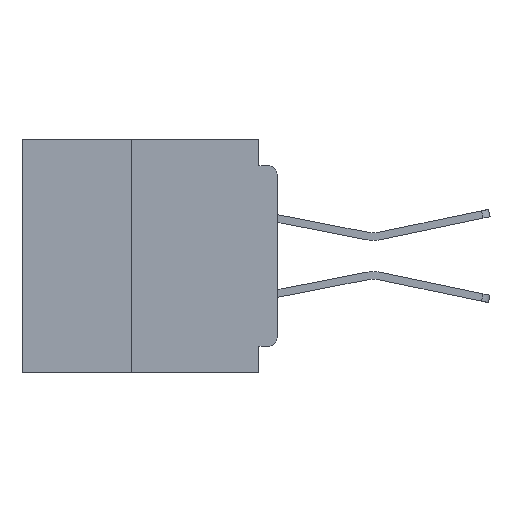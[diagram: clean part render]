
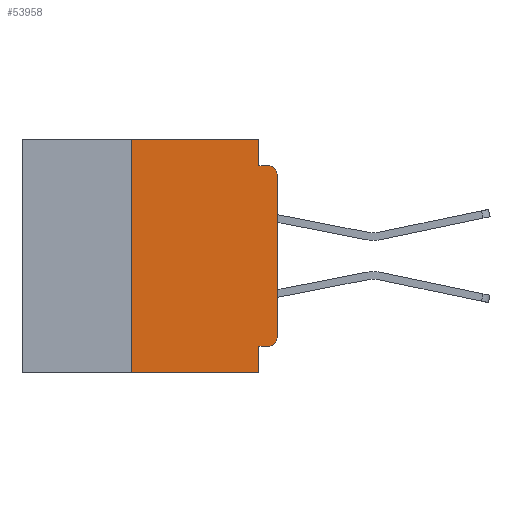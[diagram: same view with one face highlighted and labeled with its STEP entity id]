
A CAD part, left-side view. The second image highlights one B-rep face of the part: STEP entity #53958.
In plain terms, the highlighted planar face has unit normal (-1, 0, 0).
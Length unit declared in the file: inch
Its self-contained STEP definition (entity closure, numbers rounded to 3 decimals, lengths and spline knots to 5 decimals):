
#474 = AXIS2_PLACEMENT_3D ( 'NONE', #16788, #7421, #53741 ) ;
#2796 = DIRECTION ( 'NONE',  ( 0., 0., 1. ) ) ;
#4059 = DIRECTION ( 'NONE',  ( 0., 0., -1. ) ) ;
#4102 = CIRCLE ( 'NONE', #54483, 0.015 ) ;
#4127 = DIRECTION ( 'NONE',  ( 0., 0., -1. ) ) ;
#4314 = CARTESIAN_POINT ( 'NONE',  ( 0., 0., -0.34 ) ) ;
#4541 = VERTEX_POINT ( 'NONE', #58843 ) ;
#5620 = EDGE_CURVE ( 'NONE', #8508, #4541, #50075, .T. ) ;
#7166 = DIRECTION ( 'NONE',  ( 0., -1., 0. ) ) ;
#7342 = AXIS2_PLACEMENT_3D ( 'NONE', #19513, #51830, #24227 ) ;
#7421 = DIRECTION ( 'NONE',  ( 1., 0., 0. ) ) ;
#8508 = VERTEX_POINT ( 'NONE', #32192 ) ;
#8620 = VECTOR ( 'NONE', #14766, 39.37008 ) ;
#10069 = CARTESIAN_POINT ( 'NONE',  ( 0., 0.437, 0. ) ) ;
#11432 = ORIENTED_EDGE ( 'NONE', *, *, #44101, .F. ) ;
#11876 = EDGE_CURVE ( 'NONE', #43493, #4541, #48080, .T. ) ;
#14766 = DIRECTION ( 'NONE',  ( 0., -1., 0. ) ) ;
#15883 = CARTESIAN_POINT ( 'NONE',  ( 0., 0., 0. ) ) ;
#16788 = CARTESIAN_POINT ( 'NONE',  ( 0., 0.437, 0. ) ) ;
#16813 = VERTEX_POINT ( 'NONE', #34331 ) ;
#17092 = VERTEX_POINT ( 'NONE', #54370 ) ;
#17467 = LINE ( 'NONE', #44117, #40686 ) ;
#18186 = ORIENTED_EDGE ( 'NONE', *, *, #54024, .F. ) ;
#19257 = CARTESIAN_POINT ( 'NONE',  ( 0., 0.25, 0. ) ) ;
#19502 = ORIENTED_EDGE ( 'NONE', *, *, #53316, .F. ) ;
#19513 = CARTESIAN_POINT ( 'NONE',  ( 0., 0.015, -0.06 ) ) ;
#21509 = PLANE ( 'NONE',  #474 ) ;
#23134 = EDGE_CURVE ( 'NONE', #50989, #37620, #52724, .T. ) ;
#23238 = CARTESIAN_POINT ( 'NONE',  ( 0., 0., -0.355 ) ) ;
#23543 = VECTOR ( 'NONE', #4127, 39.37008 ) ;
#23968 = VECTOR ( 'NONE', #2796, 39.37008 ) ;
#24227 = DIRECTION ( 'NONE',  ( 0., 0., -1. ) ) ;
#25121 = EDGE_CURVE ( 'NONE', #17092, #43493, #39551, .T. ) ;
#25372 = ORIENTED_EDGE ( 'NONE', *, *, #23134, .T. ) ;
#26047 = CARTESIAN_POINT ( 'NONE',  ( 0., 0.25, -0.4 ) ) ;
#26382 = DIRECTION ( 'NONE',  ( 0., -1., 0. ) ) ;
#30389 = CARTESIAN_POINT ( 'NONE',  ( 0., 0.437, -0.4 ) ) ;
#31646 = VERTEX_POINT ( 'NONE', #19257 ) ;
#31930 = DIRECTION ( 'NONE',  ( -1., 0., 0. ) ) ;
#32192 = CARTESIAN_POINT ( 'NONE',  ( 0., 0.25, -0.4 ) ) ;
#34331 = CARTESIAN_POINT ( 'NONE',  ( 0., 0.031, 0. ) ) ;
#34405 = ORIENTED_EDGE ( 'NONE', *, *, #40597, .T. ) ;
#34906 = CARTESIAN_POINT ( 'NONE',  ( 0., 0.031, -0.355 ) ) ;
#35110 = ORIENTED_EDGE ( 'NONE', *, *, #25121, .F. ) ;
#35211 = ORIENTED_EDGE ( 'NONE', *, *, #46718, .T. ) ;
#36493 = CARTESIAN_POINT ( 'NONE',  ( 0., 0.031, -0.4 ) ) ;
#37620 = VERTEX_POINT ( 'NONE', #57906 ) ;
#37733 = LINE ( 'NONE', #26047, #23968 ) ;
#37915 = EDGE_LOOP ( 'NONE', ( #25372, #34405, #18186, #11432, #49824, #19502, #51871, #39170, #35110, #35211 ) ) ;
#38527 = VECTOR ( 'NONE', #26382, 39.37008 ) ;
#39010 = DIRECTION ( 'NONE',  ( 0., 0., 1. ) ) ;
#39170 = ORIENTED_EDGE ( 'NONE', *, *, #11876, .F. ) ;
#39551 = LINE ( 'NONE', #23238, #48875 ) ;
#39964 = LINE ( 'NONE', #40325, #38527 ) ;
#40325 = CARTESIAN_POINT ( 'NONE',  ( 0., 0., -0.045 ) ) ;
#40597 = EDGE_CURVE ( 'NONE', #37620, #44413, #44093, .T. ) ;
#40686 = VECTOR ( 'NONE', #48724, 39.37008 ) ;
#40754 = VECTOR ( 'NONE', #7166, 39.37008 ) ;
#41436 = DIRECTION ( 'NONE',  ( 0., 1., 0. ) ) ;
#43493 = VERTEX_POINT ( 'NONE', #34906 ) ;
#44093 = CIRCLE ( 'NONE', #7342, 0.015 ) ;
#44101 = EDGE_CURVE ( 'NONE', #16813, #48015, #17467, .T. ) ;
#44117 = CARTESIAN_POINT ( 'NONE',  ( 0., 0.031, 0. ) ) ;
#44413 = VERTEX_POINT ( 'NONE', #50902 ) ;
#45828 = EDGE_CURVE ( 'NONE', #31646, #16813, #59228, .T. ) ;
#46718 = EDGE_CURVE ( 'NONE', #17092, #50989, #4102, .T. ) ;
#48015 = VERTEX_POINT ( 'NONE', #59143 ) ;
#48080 = LINE ( 'NONE', #36493, #23543 ) ;
#48724 = DIRECTION ( 'NONE',  ( 0., 0., -1. ) ) ;
#48875 = VECTOR ( 'NONE', #41436, 39.37008 ) ;
#49824 = ORIENTED_EDGE ( 'NONE', *, *, #45828, .F. ) ;
#50075 = LINE ( 'NONE', #30389, #40754 ) ;
#50902 = CARTESIAN_POINT ( 'NONE',  ( 0., 0.015, -0.045 ) ) ;
#50989 = VERTEX_POINT ( 'NONE', #4314 ) ;
#51284 = VECTOR ( 'NONE', #39010, 39.37008 ) ;
#51830 = DIRECTION ( 'NONE',  ( -1., 0., 0. ) ) ;
#51871 = ORIENTED_EDGE ( 'NONE', *, *, #5620, .T. ) ;
#52724 = LINE ( 'NONE', #15883, #51284 ) ;
#53316 = EDGE_CURVE ( 'NONE', #8508, #31646, #37733, .T. ) ;
#53594 = FACE_OUTER_BOUND ( 'NONE', #37915, .T. ) ;
#53741 = DIRECTION ( 'NONE',  ( 0., 0., -1. ) ) ;
#53958 = ADVANCED_FACE ( 'NONE', ( #53594 ), #21509, .F. ) ;
#54024 = EDGE_CURVE ( 'NONE', #48015, #44413, #39964, .T. ) ;
#54370 = CARTESIAN_POINT ( 'NONE',  ( 0., 0.015, -0.355 ) ) ;
#54483 = AXIS2_PLACEMENT_3D ( 'NONE', #59475, #31930, #4059 ) ;
#57906 = CARTESIAN_POINT ( 'NONE',  ( 0., 0., -0.06 ) ) ;
#58843 = CARTESIAN_POINT ( 'NONE',  ( 0., 0.031, -0.4 ) ) ;
#59143 = CARTESIAN_POINT ( 'NONE',  ( 0., 0.031, -0.045 ) ) ;
#59228 = LINE ( 'NONE', #10069, #8620 ) ;
#59475 = CARTESIAN_POINT ( 'NONE',  ( 0., 0.015, -0.34 ) ) ;
